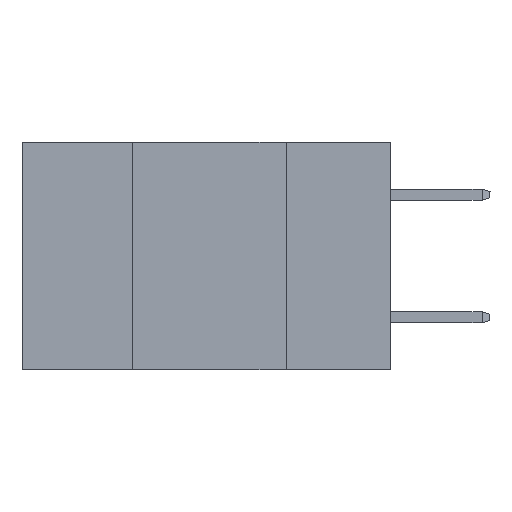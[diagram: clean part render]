
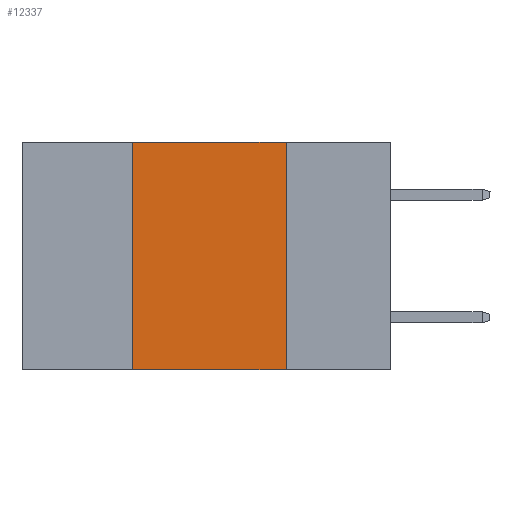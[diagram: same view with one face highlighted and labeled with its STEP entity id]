
A CAD part, left-side view. The second image highlights one B-rep face of the part: STEP entity #12337.
In plain terms, the highlighted planar face has unit normal (-1, 0, 0).
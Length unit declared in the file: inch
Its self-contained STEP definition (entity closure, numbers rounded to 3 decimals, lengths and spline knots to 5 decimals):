
#483 = DIRECTION ( 'NONE',  ( 0., 0., 1. ) ) ;
#814 = VECTOR ( 'NONE', #5717, 39.37008 ) ;
#2283 = VECTOR ( 'NONE', #21075, 39.37008 ) ;
#4197 = EDGE_CURVE ( 'NONE', #13194, #18466, #6380, .T. ) ;
#4514 = ORIENTED_EDGE ( 'NONE', *, *, #4881, .F. ) ;
#4881 = EDGE_CURVE ( 'NONE', #18466, #19128, #22349, .T. ) ;
#5264 = CARTESIAN_POINT ( 'NONE',  ( 0., 0.6, -0.37 ) ) ;
#5324 = VECTOR ( 'NONE', #15851, 39.37008 ) ;
#5696 = CARTESIAN_POINT ( 'NONE',  ( 0., 0.42, -0.37 ) ) ;
#5717 = DIRECTION ( 'NONE',  ( 0., 0., -1. ) ) ;
#5798 = PLANE ( 'NONE',  #19322 ) ;
#6380 = LINE ( 'NONE', #13734, #2283 ) ;
#8226 = CARTESIAN_POINT ( 'NONE',  ( 0., 0.42, 0. ) ) ;
#9850 = ORIENTED_EDGE ( 'NONE', *, *, #4197, .F. ) ;
#11376 = LINE ( 'NONE', #8226, #20558 ) ;
#12337 = ADVANCED_FACE ( 'NONE', ( #15179 ), #5798, .F. ) ;
#13194 = VERTEX_POINT ( 'NONE', #22496 ) ;
#13714 = CARTESIAN_POINT ( 'NONE',  ( 0., 0.17, -0.37 ) ) ;
#13734 = CARTESIAN_POINT ( 'NONE',  ( 0., 0.6, 0. ) ) ;
#14536 = EDGE_CURVE ( 'NONE', #18570, #13194, #11376, .T. ) ;
#15179 = FACE_OUTER_BOUND ( 'NONE', #20633, .T. ) ;
#15401 = ORIENTED_EDGE ( 'NONE', *, *, #19275, .T. ) ;
#15851 = DIRECTION ( 'NONE',  ( 0., -1., 0. ) ) ;
#17623 = CARTESIAN_POINT ( 'NONE',  ( 0., 0.17, 0. ) ) ;
#18466 = VERTEX_POINT ( 'NONE', #17623 ) ;
#18570 = VERTEX_POINT ( 'NONE', #5696 ) ;
#19128 = VERTEX_POINT ( 'NONE', #13714 ) ;
#19275 = EDGE_CURVE ( 'NONE', #18570, #19128, #23699, .T. ) ;
#19322 = AXIS2_PLACEMENT_3D ( 'NONE', #22554, #22430, #20726 ) ;
#20558 = VECTOR ( 'NONE', #483, 39.37008 ) ;
#20633 = EDGE_LOOP ( 'NONE', ( #4514, #9850, #20715, #15401 ) ) ;
#20715 = ORIENTED_EDGE ( 'NONE', *, *, #14536, .F. ) ;
#20726 = DIRECTION ( 'NONE',  ( 0., 0., -1. ) ) ;
#21075 = DIRECTION ( 'NONE',  ( 0., -1., 0. ) ) ;
#22238 = CARTESIAN_POINT ( 'NONE',  ( 0., 0.17, 0. ) ) ;
#22349 = LINE ( 'NONE', #22238, #814 ) ;
#22430 = DIRECTION ( 'NONE',  ( 1., 0., 0. ) ) ;
#22496 = CARTESIAN_POINT ( 'NONE',  ( 0., 0.42, 0. ) ) ;
#22554 = CARTESIAN_POINT ( 'NONE',  ( 0., 0.6, 0. ) ) ;
#23699 = LINE ( 'NONE', #5264, #5324 ) ;
